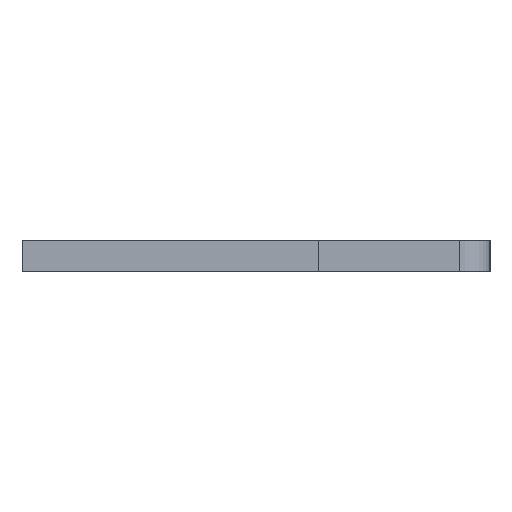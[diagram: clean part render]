
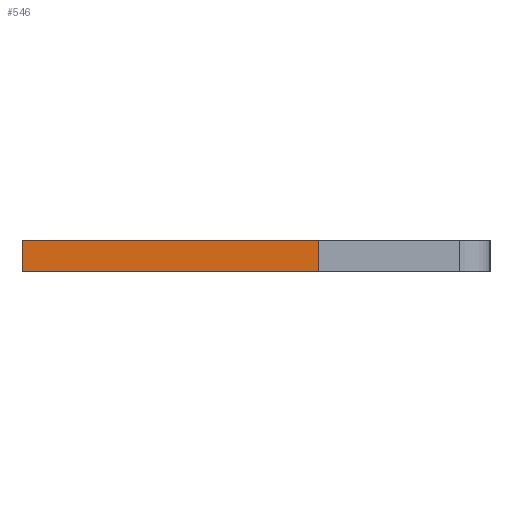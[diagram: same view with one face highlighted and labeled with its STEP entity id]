
A CAD part, left-side view. The second image highlights one B-rep face of the part: STEP entity #546.
In plain terms, the highlighted face is planar.
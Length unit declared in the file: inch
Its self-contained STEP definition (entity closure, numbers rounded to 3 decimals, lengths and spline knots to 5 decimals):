
#19 = ORIENTED_EDGE ( 'NONE', *, *, #974, .T. ) ;
#56 = EDGE_CURVE ( 'NONE', #924, #780, #942, .T. ) ;
#244 = PLANE ( 'NONE',  #920 ) ;
#296 = VERTEX_POINT ( 'NONE', #750 ) ;
#332 = VECTOR ( 'NONE', #363, 39.37008 ) ;
#363 = DIRECTION ( 'NONE',  ( -1., 0., 0. ) ) ;
#422 = CARTESIAN_POINT ( 'NONE',  ( -0.01, 0.15, -0.04 ) ) ;
#453 = ORIENTED_EDGE ( 'NONE', *, *, #1049, .F. ) ;
#517 = FACE_OUTER_BOUND ( 'NONE', #1472, .T. ) ;
#546 = ADVANCED_FACE ( 'NONE', ( #517 ), #244, .F. ) ;
#550 = DIRECTION ( 'NONE',  ( -1., 0., 0. ) ) ;
#556 = CARTESIAN_POINT ( 'NONE',  ( 0.01, -0.04, -0.04 ) ) ;
#656 = VECTOR ( 'NONE', #1387, 39.37008 ) ;
#750 = CARTESIAN_POINT ( 'NONE',  ( -0.01, -0.04, -0.04 ) ) ;
#763 = DIRECTION ( 'NONE',  ( 0., 0., 1. ) ) ;
#773 = CARTESIAN_POINT ( 'NONE',  ( 0.01, 0.15, -0.04 ) ) ;
#780 = VERTEX_POINT ( 'NONE', #1180 ) ;
#827 = DIRECTION ( 'NONE',  ( 0., 1., 0. ) ) ;
#877 = VECTOR ( 'NONE', #550, 39.37008 ) ;
#920 = AXIS2_PLACEMENT_3D ( 'NONE', #773, #763, #1734 ) ;
#924 = VERTEX_POINT ( 'NONE', #556 ) ;
#925 = LINE ( 'NONE', #1510, #877 ) ;
#942 = LINE ( 'NONE', #1447, #656 ) ;
#974 = EDGE_CURVE ( 'NONE', #296, #1509, #1665, .T. ) ;
#1028 = LINE ( 'NONE', #1069, #332 ) ;
#1049 = EDGE_CURVE ( 'NONE', #780, #1509, #925, .T. ) ;
#1069 = CARTESIAN_POINT ( 'NONE',  ( 0.01, -0.04, -0.04 ) ) ;
#1180 = CARTESIAN_POINT ( 'NONE',  ( 0.01, 0.15, -0.04 ) ) ;
#1194 = VECTOR ( 'NONE', #827, 39.37008 ) ;
#1387 = DIRECTION ( 'NONE',  ( 0., 1., 0. ) ) ;
#1447 = CARTESIAN_POINT ( 'NONE',  ( 0.01, 0.15, -0.04 ) ) ;
#1472 = EDGE_LOOP ( 'NONE', ( #19, #453, #1711, #1478 ) ) ;
#1478 = ORIENTED_EDGE ( 'NONE', *, *, #1659, .T. ) ;
#1509 = VERTEX_POINT ( 'NONE', #1732 ) ;
#1510 = CARTESIAN_POINT ( 'NONE',  ( 0.01, 0.15, -0.04 ) ) ;
#1659 = EDGE_CURVE ( 'NONE', #924, #296, #1028, .T. ) ;
#1665 = LINE ( 'NONE', #422, #1194 ) ;
#1711 = ORIENTED_EDGE ( 'NONE', *, *, #56, .F. ) ;
#1732 = CARTESIAN_POINT ( 'NONE',  ( -0.01, 0.15, -0.04 ) ) ;
#1734 = DIRECTION ( 'NONE',  ( 1., 0., 0. ) ) ;
